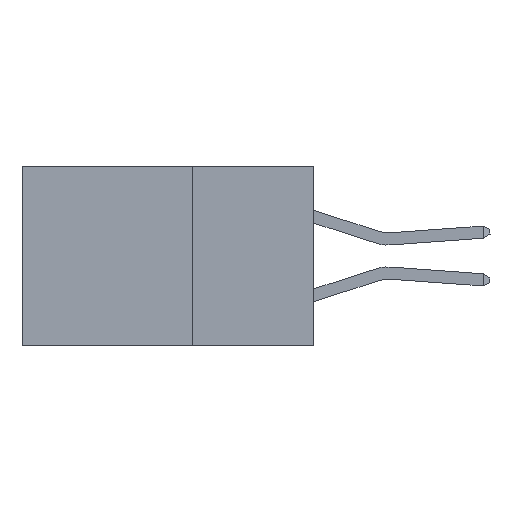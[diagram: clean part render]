
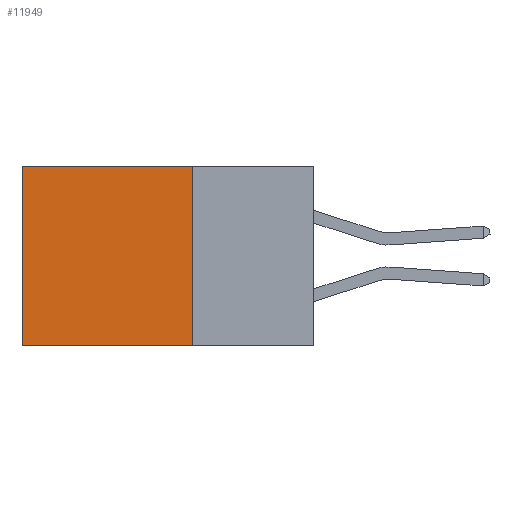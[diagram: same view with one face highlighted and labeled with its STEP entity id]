
A CAD part, left-side view. The second image highlights one B-rep face of the part: STEP entity #11949.
In plain terms, the highlighted planar face has unit normal (-1, 0, 0).
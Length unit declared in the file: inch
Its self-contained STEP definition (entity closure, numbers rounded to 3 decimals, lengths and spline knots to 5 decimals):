
#3408 = CARTESIAN_POINT ( 'NONE',  ( 0.2875, 0.25, 0. ) ) ;
#5842 = EDGE_CURVE ( 'NONE', #31438, #19037, #24197, .T. ) ;
#6028 = CARTESIAN_POINT ( 'NONE',  ( 0.2875, 0.25, 0. ) ) ;
#7264 = VECTOR ( 'NONE', #22403, 39.37008 ) ;
#7787 = EDGE_CURVE ( 'NONE', #31438, #20274, #20789, .T. ) ;
#7910 = ORIENTED_EDGE ( 'NONE', *, *, #7787, .T. ) ;
#8826 = PLANE ( 'NONE',  #12328 ) ;
#11406 = CARTESIAN_POINT ( 'NONE',  ( 0.2875, 0.25, 0. ) ) ;
#11594 = DIRECTION ( 'NONE',  ( 0., 0., -1. ) ) ;
#11949 = ADVANCED_FACE ( 'NONE', ( #15806 ), #8826, .F. ) ;
#12328 = AXIS2_PLACEMENT_3D ( 'NONE', #6028, #27445, #11594 ) ;
#12543 = CARTESIAN_POINT ( 'NONE',  ( 0.2875, 0.25, 0. ) ) ;
#15806 = FACE_OUTER_BOUND ( 'NONE', #28674, .T. ) ;
#16212 = ORIENTED_EDGE ( 'NONE', *, *, #23045, .F. ) ;
#18271 = CARTESIAN_POINT ( 'NONE',  ( 0.2875, 0.25, -0.37 ) ) ;
#18718 = ORIENTED_EDGE ( 'NONE', *, *, #20697, .T. ) ;
#19037 = VERTEX_POINT ( 'NONE', #18271 ) ;
#19205 = ORIENTED_EDGE ( 'NONE', *, *, #5842, .F. ) ;
#19494 = DIRECTION ( 'NONE',  ( 0., 0., -1. ) ) ;
#19843 = VERTEX_POINT ( 'NONE', #31874 ) ;
#20274 = VERTEX_POINT ( 'NONE', #22814 ) ;
#20697 = EDGE_CURVE ( 'NONE', #20274, #19843, #22205, .T. ) ;
#20789 = LINE ( 'NONE', #3408, #7264 ) ;
#21823 = DIRECTION ( 'NONE',  ( 0., 1., 0. ) ) ;
#22205 = LINE ( 'NONE', #24286, #28329 ) ;
#22403 = DIRECTION ( 'NONE',  ( 0., 1., 0. ) ) ;
#22814 = CARTESIAN_POINT ( 'NONE',  ( 0.2875, 0.6, 0. ) ) ;
#23045 = EDGE_CURVE ( 'NONE', #19037, #19843, #26898, .T. ) ;
#24197 = LINE ( 'NONE', #11406, #29514 ) ;
#24286 = CARTESIAN_POINT ( 'NONE',  ( 0.2875, 0.6, 0. ) ) ;
#24435 = CARTESIAN_POINT ( 'NONE',  ( 0.2875, 0.25, -0.37 ) ) ;
#26079 = VECTOR ( 'NONE', #21823, 39.37008 ) ;
#26898 = LINE ( 'NONE', #24435, #26079 ) ;
#27445 = DIRECTION ( 'NONE',  ( 1., 0., 0. ) ) ;
#28329 = VECTOR ( 'NONE', #32211, 39.37008 ) ;
#28674 = EDGE_LOOP ( 'NONE', ( #18718, #16212, #19205, #7910 ) ) ;
#29514 = VECTOR ( 'NONE', #19494, 39.37008 ) ;
#31438 = VERTEX_POINT ( 'NONE', #12543 ) ;
#31874 = CARTESIAN_POINT ( 'NONE',  ( 0.2875, 0.6, -0.37 ) ) ;
#32211 = DIRECTION ( 'NONE',  ( 0., 0., -1. ) ) ;
